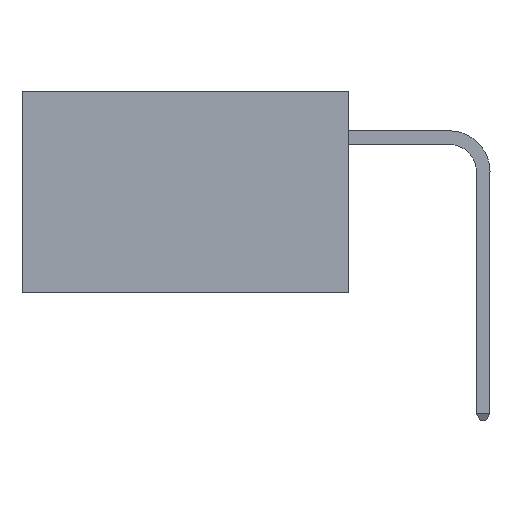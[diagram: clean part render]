
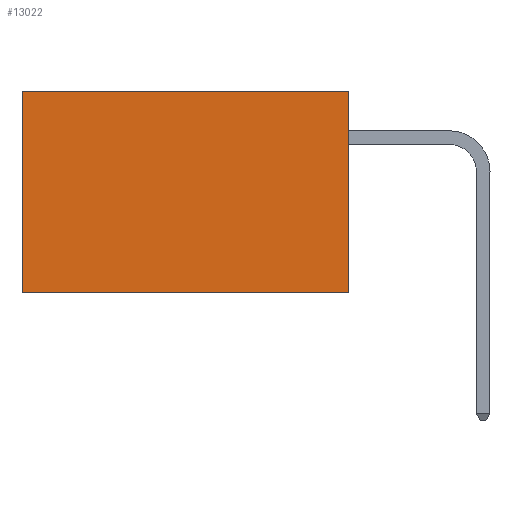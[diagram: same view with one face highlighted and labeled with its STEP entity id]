
A CAD part, left-side view. The second image highlights one B-rep face of the part: STEP entity #13022.
In plain terms, the highlighted planar face has unit normal (-1, 0, 0).
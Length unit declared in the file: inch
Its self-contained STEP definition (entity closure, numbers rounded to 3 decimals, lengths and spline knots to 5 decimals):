
#37 = ORIENTED_EDGE ( 'NONE', *, *, #316, .F. ) ;
#316 = EDGE_CURVE ( 'NONE', #8680, #6655, #9014, .T. ) ;
#773 = EDGE_LOOP ( 'NONE', ( #5500, #8119, #37, #11939 ) ) ;
#805 = CARTESIAN_POINT ( 'NONE',  ( 0.2875, 0., -0.37 ) ) ;
#1617 = CARTESIAN_POINT ( 'NONE',  ( 0.2875, 0.6, -0.37 ) ) ;
#2003 = CARTESIAN_POINT ( 'NONE',  ( 0.2875, 0., 0. ) ) ;
#2085 = LINE ( 'NONE', #8525, #12677 ) ;
#2311 = LINE ( 'NONE', #7068, #10364 ) ;
#2793 = VERTEX_POINT ( 'NONE', #1617 ) ;
#3152 = DIRECTION ( 'NONE',  ( 1., 0., 0. ) ) ;
#5492 = FACE_OUTER_BOUND ( 'NONE', #773, .T. ) ;
#5500 = ORIENTED_EDGE ( 'NONE', *, *, #12504, .T. ) ;
#5585 = EDGE_CURVE ( 'NONE', #6655, #2793, #10499, .T. ) ;
#5882 = DIRECTION ( 'NONE',  ( 0., 0., -1. ) ) ;
#6276 = VERTEX_POINT ( 'NONE', #7801 ) ;
#6655 = VERTEX_POINT ( 'NONE', #805 ) ;
#7068 = CARTESIAN_POINT ( 'NONE',  ( 0.2875, 0., 0. ) ) ;
#7801 = CARTESIAN_POINT ( 'NONE',  ( 0.2875, 0.6, 0. ) ) ;
#8079 = DIRECTION ( 'NONE',  ( 0., 1., 0. ) ) ;
#8119 = ORIENTED_EDGE ( 'NONE', *, *, #5585, .F. ) ;
#8525 = CARTESIAN_POINT ( 'NONE',  ( 0.2875, 0.6, 0. ) ) ;
#8680 = VERTEX_POINT ( 'NONE', #11699 ) ;
#9014 = LINE ( 'NONE', #12227, #9320 ) ;
#9320 = VECTOR ( 'NONE', #5882, 39.37008 ) ;
#9550 = DIRECTION ( 'NONE',  ( 0., 0., -1. ) ) ;
#10266 = DIRECTION ( 'NONE',  ( 0., 1., 0. ) ) ;
#10364 = VECTOR ( 'NONE', #8079, 39.37008 ) ;
#10426 = DIRECTION ( 'NONE',  ( 0., 0., -1. ) ) ;
#10499 = LINE ( 'NONE', #12586, #12702 ) ;
#10649 = EDGE_CURVE ( 'NONE', #8680, #6276, #2311, .T. ) ;
#10828 = AXIS2_PLACEMENT_3D ( 'NONE', #2003, #3152, #10426 ) ;
#11699 = CARTESIAN_POINT ( 'NONE',  ( 0.2875, 0., 0. ) ) ;
#11939 = ORIENTED_EDGE ( 'NONE', *, *, #10649, .T. ) ;
#12227 = CARTESIAN_POINT ( 'NONE',  ( 0.2875, 0., 0. ) ) ;
#12504 = EDGE_CURVE ( 'NONE', #6276, #2793, #2085, .T. ) ;
#12586 = CARTESIAN_POINT ( 'NONE',  ( 0.2875, 0., -0.37 ) ) ;
#12677 = VECTOR ( 'NONE', #9550, 39.37008 ) ;
#12702 = VECTOR ( 'NONE', #10266, 39.37008 ) ;
#13022 = ADVANCED_FACE ( 'NONE', ( #5492 ), #13221, .F. ) ;
#13221 = PLANE ( 'NONE',  #10828 ) ;
